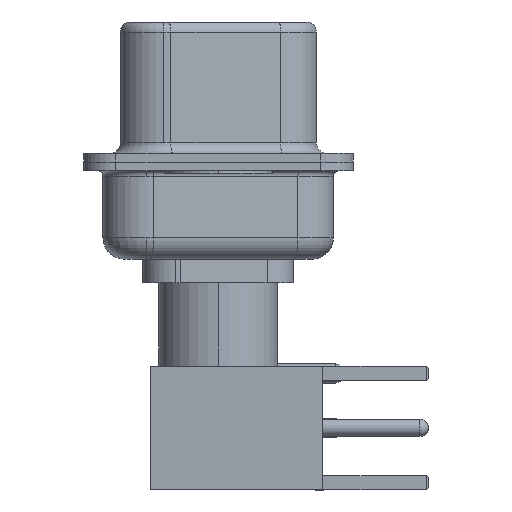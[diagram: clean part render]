
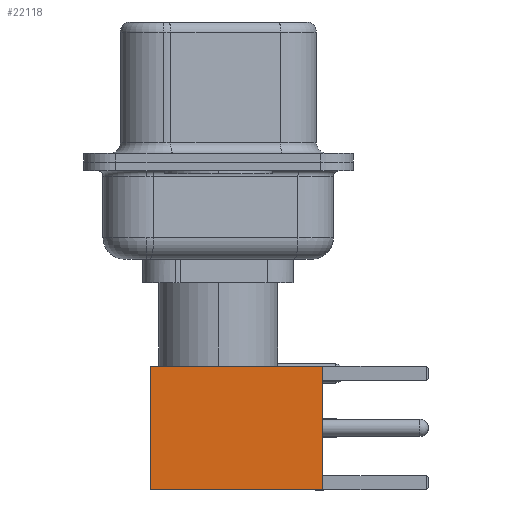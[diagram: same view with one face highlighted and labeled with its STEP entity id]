
A CAD part, left-side view. The second image highlights one B-rep face of the part: STEP entity #22118.
In plain terms, the highlighted face is planar.
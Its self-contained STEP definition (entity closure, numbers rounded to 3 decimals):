
#473 = VECTOR ( 'NONE', #23338, 1000. ) ;
#2762 = EDGE_CURVE ( 'NONE', #28229, #12869, #30083, .T. ) ;
#3680 = VERTEX_POINT ( 'NONE', #28447 ) ;
#4770 = DIRECTION ( 'NONE',  ( 0., 0., -1. ) ) ;
#7826 = AXIS2_PLACEMENT_3D ( 'NONE', #16874, #23937, #28813 ) ;
#8260 = DIRECTION ( 'NONE',  ( -1., 0., 0. ) ) ;
#8275 = EDGE_CURVE ( 'NONE', #3680, #28229, #18154, .T. ) ;
#9071 = ORIENTED_EDGE ( 'NONE', *, *, #27101, .F. ) ;
#9174 = CARTESIAN_POINT ( 'NONE',  ( 2.875, 2.875, 0. ) ) ;
#9705 = VERTEX_POINT ( 'NONE', #16892 ) ;
#10346 = LINE ( 'NONE', #25673, #473 ) ;
#10537 = ORIENTED_EDGE ( 'NONE', *, *, #24360, .F. ) ;
#10957 = VECTOR ( 'NONE', #8260, 1000. ) ;
#11512 = PLANE ( 'NONE',  #7826 ) ;
#12456 = EDGE_LOOP ( 'NONE', ( #30138, #26996, #9071, #10537 ) ) ;
#12869 = VERTEX_POINT ( 'NONE', #25731 ) ;
#14210 = VECTOR ( 'NONE', #4770, 1000. ) ;
#14515 = CARTESIAN_POINT ( 'NONE',  ( -2.875, 2.875, 0. ) ) ;
#15336 = CARTESIAN_POINT ( 'NONE',  ( 0., 2.875, 0. ) ) ;
#16566 = FACE_OUTER_BOUND ( 'NONE', #12456, .T. ) ;
#16864 = LINE ( 'NONE', #14515, #14210 ) ;
#16874 = CARTESIAN_POINT ( 'NONE',  ( 2.875, 2.875, 0. ) ) ;
#16892 = CARTESIAN_POINT ( 'NONE',  ( -2.875, 2.875, 8. ) ) ;
#18154 = LINE ( 'NONE', #29919, #29850 ) ;
#22118 = ADVANCED_FACE ( 'NONE', ( #16566 ), #11512, .T. ) ;
#23338 = DIRECTION ( 'NONE',  ( -1., 0., 0. ) ) ;
#23937 = DIRECTION ( 'NONE',  ( 0., 1., 0. ) ) ;
#24360 = EDGE_CURVE ( 'NONE', #3680, #9705, #10346, .T. ) ;
#25053 = DIRECTION ( 'NONE',  ( 0., 0., -1. ) ) ;
#25673 = CARTESIAN_POINT ( 'NONE',  ( 0., 2.875, 8. ) ) ;
#25731 = CARTESIAN_POINT ( 'NONE',  ( -2.875, 2.875, 0. ) ) ;
#26996 = ORIENTED_EDGE ( 'NONE', *, *, #2762, .T. ) ;
#27101 = EDGE_CURVE ( 'NONE', #9705, #12869, #16864, .T. ) ;
#28229 = VERTEX_POINT ( 'NONE', #9174 ) ;
#28447 = CARTESIAN_POINT ( 'NONE',  ( 2.875, 2.875, 8. ) ) ;
#28813 = DIRECTION ( 'NONE',  ( 0., 0., 1. ) ) ;
#29850 = VECTOR ( 'NONE', #25053, 1000. ) ;
#29919 = CARTESIAN_POINT ( 'NONE',  ( 2.875, 2.875, 0. ) ) ;
#30083 = LINE ( 'NONE', #15336, #10957 ) ;
#30138 = ORIENTED_EDGE ( 'NONE', *, *, #8275, .T. ) ;
